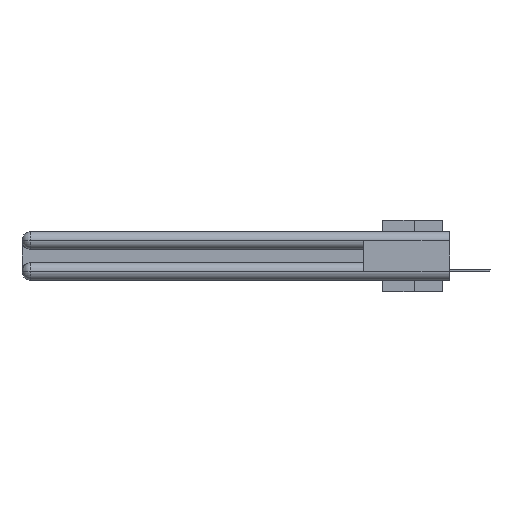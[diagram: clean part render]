
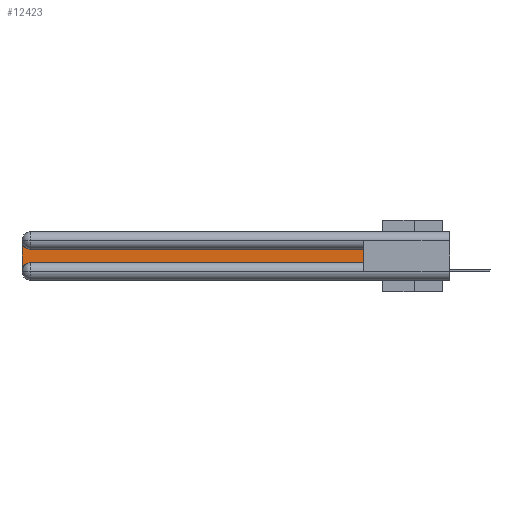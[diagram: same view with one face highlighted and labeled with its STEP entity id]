
A CAD part, left-side view. The second image highlights one B-rep face of the part: STEP entity #12423.
In plain terms, the highlighted planar face has unit normal (-1, 0, 0).
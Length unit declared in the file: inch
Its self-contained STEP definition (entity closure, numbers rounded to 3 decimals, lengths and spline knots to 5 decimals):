
#624 = ORIENTED_EDGE ( 'NONE', *, *, #15332, .T. ) ;
#962 = EDGE_CURVE ( 'NONE', #19508, #28716, #30767, .T. ) ;
#1839 = DIRECTION ( 'NONE',  ( 1., 0., 0. ) ) ;
#1992 = CARTESIAN_POINT ( 'NONE',  ( 0.075, 0.6, -0.2175 ) ) ;
#2482 = CARTESIAN_POINT ( 'NONE',  ( 0.075, 3., -0.0625 ) ) ;
#4892 = DIRECTION ( 'NONE',  ( 0., 0., -1. ) ) ;
#4906 = CARTESIAN_POINT ( 'NONE',  ( 0.075, 3., -0.2175 ) ) ;
#5218 = ORIENTED_EDGE ( 'NONE', *, *, #29994, .T. ) ;
#5358 = VECTOR ( 'NONE', #18011, 39.37008 ) ;
#6197 = CIRCLE ( 'NONE', #20833, 0.06 ) ;
#7261 = PLANE ( 'NONE',  #29464 ) ;
#7985 = ORIENTED_EDGE ( 'NONE', *, *, #10760, .T. ) ;
#8888 = CARTESIAN_POINT ( 'NONE',  ( 0.075, 0.6, -0.1225 ) ) ;
#9007 = CARTESIAN_POINT ( 'NONE',  ( 0.075, 3., -0.2775 ) ) ;
#9601 = FACE_OUTER_BOUND ( 'NONE', #22230, .T. ) ;
#10035 = AXIS2_PLACEMENT_3D ( 'NONE', #25823, #27752, #13176 ) ;
#10313 = VECTOR ( 'NONE', #16152, 39.37008 ) ;
#10516 = CARTESIAN_POINT ( 'NONE',  ( 0.075, 2.94, -0.1225 ) ) ;
#10735 = CARTESIAN_POINT ( 'NONE',  ( 0.075, 0.6, -0.2175 ) ) ;
#10760 = EDGE_CURVE ( 'NONE', #24256, #14209, #6197, .T. ) ;
#11482 = VECTOR ( 'NONE', #12153, 39.37008 ) ;
#12153 = DIRECTION ( 'NONE',  ( 0., 0., -1. ) ) ;
#12423 = ADVANCED_FACE ( 'NONE', ( #9601 ), #7261, .F. ) ;
#13176 = DIRECTION ( 'NONE',  ( 0., 0., -1. ) ) ;
#13858 = ORIENTED_EDGE ( 'NONE', *, *, #26111, .T. ) ;
#14209 = VERTEX_POINT ( 'NONE', #2482 ) ;
#15332 = EDGE_CURVE ( 'NONE', #28716, #29244, #18627, .T. ) ;
#16152 = DIRECTION ( 'NONE',  ( 0., 1., 0. ) ) ;
#16245 = CARTESIAN_POINT ( 'NONE',  ( 0.075, 0.6, -0.1225 ) ) ;
#16453 = VERTEX_POINT ( 'NONE', #16245 ) ;
#16870 = CARTESIAN_POINT ( 'NONE',  ( 0.075, 3., -0.1225 ) ) ;
#16889 = LINE ( 'NONE', #4906, #11482 ) ;
#17890 = EDGE_CURVE ( 'NONE', #14209, #19508, #16889, .T. ) ;
#18011 = DIRECTION ( 'NONE',  ( 0., -1., 0. ) ) ;
#18299 = CARTESIAN_POINT ( 'NONE',  ( 0.075, 2.94, -0.2175 ) ) ;
#18627 = LINE ( 'NONE', #10735, #5358 ) ;
#19508 = VERTEX_POINT ( 'NONE', #9007 ) ;
#20833 = AXIS2_PLACEMENT_3D ( 'NONE', #21285, #1839, #28430 ) ;
#21285 = CARTESIAN_POINT ( 'NONE',  ( 0.075, 2.94, -0.0625 ) ) ;
#22230 = EDGE_LOOP ( 'NONE', ( #13858, #7985, #25053, #26685, #624, #5218 ) ) ;
#23376 = DIRECTION ( 'NONE',  ( 0., 0., 1. ) ) ;
#24256 = VERTEX_POINT ( 'NONE', #10516 ) ;
#25053 = ORIENTED_EDGE ( 'NONE', *, *, #17890, .T. ) ;
#25434 = LINE ( 'NONE', #26068, #30122 ) ;
#25823 = CARTESIAN_POINT ( 'NONE',  ( 0.075, 2.94, -0.2775 ) ) ;
#26068 = CARTESIAN_POINT ( 'NONE',  ( 0.075, 0.6, -0.2175 ) ) ;
#26111 = EDGE_CURVE ( 'NONE', #16453, #24256, #30447, .T. ) ;
#26549 = DIRECTION ( 'NONE',  ( 1., 0., 0. ) ) ;
#26685 = ORIENTED_EDGE ( 'NONE', *, *, #962, .T. ) ;
#27752 = DIRECTION ( 'NONE',  ( 1., 0., 0. ) ) ;
#28430 = DIRECTION ( 'NONE',  ( 0., 0., -1. ) ) ;
#28716 = VERTEX_POINT ( 'NONE', #18299 ) ;
#29244 = VERTEX_POINT ( 'NONE', #1992 ) ;
#29464 = AXIS2_PLACEMENT_3D ( 'NONE', #16870, #26549, #4892 ) ;
#29994 = EDGE_CURVE ( 'NONE', #29244, #16453, #25434, .T. ) ;
#30122 = VECTOR ( 'NONE', #23376, 39.37008 ) ;
#30447 = LINE ( 'NONE', #8888, #10313 ) ;
#30767 = CIRCLE ( 'NONE', #10035, 0.06 ) ;
